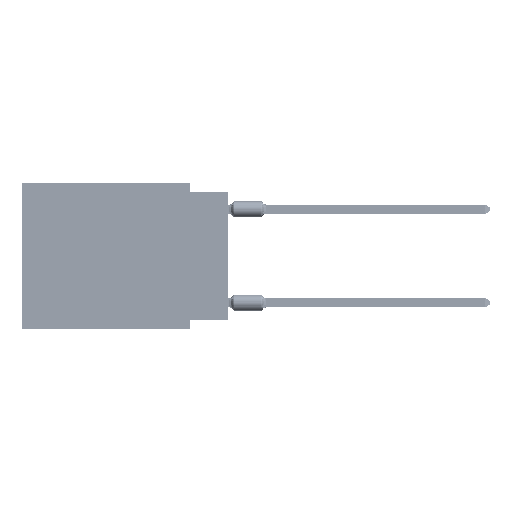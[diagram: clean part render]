
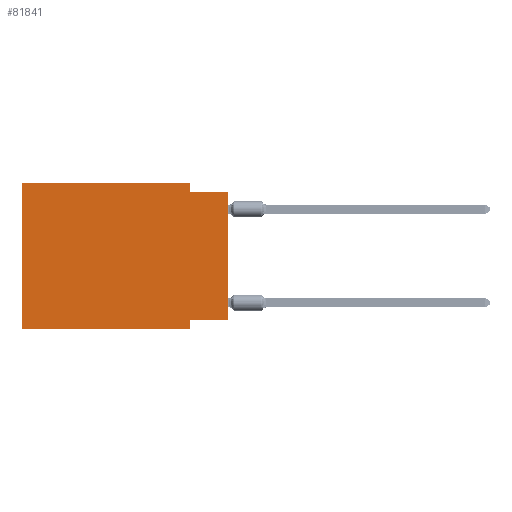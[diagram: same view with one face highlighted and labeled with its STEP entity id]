
A CAD part, left-side view. The second image highlights one B-rep face of the part: STEP entity #81841.
In plain terms, the highlighted planar face has unit normal (-1, 0, 0).
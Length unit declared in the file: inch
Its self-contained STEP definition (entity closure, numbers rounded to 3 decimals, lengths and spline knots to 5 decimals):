
#210 = LINE ( 'NONE', #67478, #28942 ) ;
#4783 = CARTESIAN_POINT ( 'NONE',  ( 0., 0.1, 0. ) ) ;
#5134 = EDGE_CURVE ( 'NONE', #66802, #17737, #49236, .T. ) ;
#6592 = DIRECTION ( 'NONE',  ( 0., 0., -1. ) ) ;
#6637 = VECTOR ( 'NONE', #6592, 39.37008 ) ;
#8726 = VERTEX_POINT ( 'NONE', #70090 ) ;
#9835 = AXIS2_PLACEMENT_3D ( 'NONE', #36340, #56525, #29174 ) ;
#14161 = DIRECTION ( 'NONE',  ( 0., -1., 0. ) ) ;
#15263 = FACE_OUTER_BOUND ( 'NONE', #15347, .T. ) ;
#15347 = EDGE_LOOP ( 'NONE', ( #36349, #33733, #61894, #77230, #71015, #83137, #86440, #34838 ) ) ;
#16062 = VERTEX_POINT ( 'NONE', #21957 ) ;
#17737 = VERTEX_POINT ( 'NONE', #36711 ) ;
#17960 = LINE ( 'NONE', #51176, #39999 ) ;
#20198 = DIRECTION ( 'NONE',  ( 0., -1., 0. ) ) ;
#20569 = CARTESIAN_POINT ( 'NONE',  ( 0., 0., -0.365 ) ) ;
#21957 = CARTESIAN_POINT ( 'NONE',  ( 0., 0., -0.365 ) ) ;
#26062 = LINE ( 'NONE', #67277, #36022 ) ;
#28281 = VECTOR ( 'NONE', #14161, 39.37008 ) ;
#28587 = DIRECTION ( 'NONE',  ( 0., 0., 1. ) ) ;
#28942 = VECTOR ( 'NONE', #47772, 39.37008 ) ;
#29174 = DIRECTION ( 'NONE',  ( 0., 0., -1. ) ) ;
#31459 = VERTEX_POINT ( 'NONE', #50695 ) ;
#32402 = CARTESIAN_POINT ( 'NONE',  ( 0., 0., -0.025 ) ) ;
#33261 = EDGE_CURVE ( 'NONE', #17737, #31459, #67974, .T. ) ;
#33515 = VERTEX_POINT ( 'NONE', #32402 ) ;
#33733 = ORIENTED_EDGE ( 'NONE', *, *, #40200, .F. ) ;
#34273 = CARTESIAN_POINT ( 'NONE',  ( 0., 0.55, -0.39 ) ) ;
#34436 = CARTESIAN_POINT ( 'NONE',  ( 0., 0.1, -0.39 ) ) ;
#34838 = ORIENTED_EDGE ( 'NONE', *, *, #75110, .F. ) ;
#36022 = VECTOR ( 'NONE', #20198, 39.37008 ) ;
#36340 = CARTESIAN_POINT ( 'NONE',  ( 0., 0.55, 0. ) ) ;
#36349 = ORIENTED_EDGE ( 'NONE', *, *, #38085, .T. ) ;
#36711 = CARTESIAN_POINT ( 'NONE',  ( 0., 0.55, 0. ) ) ;
#38085 = EDGE_CURVE ( 'NONE', #16062, #33515, #210, .T. ) ;
#39011 = CARTESIAN_POINT ( 'NONE',  ( 0., 0.1, -0.025 ) ) ;
#39999 = VECTOR ( 'NONE', #87417, 39.37008 ) ;
#40200 = EDGE_CURVE ( 'NONE', #45737, #33515, #26062, .T. ) ;
#44770 = DIRECTION ( 'NONE',  ( 0., 0., -1. ) ) ;
#45737 = VERTEX_POINT ( 'NONE', #39011 ) ;
#47772 = DIRECTION ( 'NONE',  ( 0., 0., 1. ) ) ;
#48720 = CARTESIAN_POINT ( 'NONE',  ( 0., 0.55, 0. ) ) ;
#49236 = LINE ( 'NONE', #76986, #67402 ) ;
#50695 = CARTESIAN_POINT ( 'NONE',  ( 0., 0.1, 0. ) ) ;
#51176 = CARTESIAN_POINT ( 'NONE',  ( 0., 0.55, -0.39 ) ) ;
#52433 = EDGE_CURVE ( 'NONE', #75968, #8726, #55484, .T. ) ;
#55484 = LINE ( 'NONE', #34436, #6637 ) ;
#56525 = DIRECTION ( 'NONE',  ( 1., 0., 0. ) ) ;
#56612 = VECTOR ( 'NONE', #44770, 39.37008 ) ;
#57288 = EDGE_CURVE ( 'NONE', #66802, #8726, #17960, .T. ) ;
#60546 = LINE ( 'NONE', #20569, #72270 ) ;
#61756 = EDGE_CURVE ( 'NONE', #31459, #45737, #66237, .T. ) ;
#61894 = ORIENTED_EDGE ( 'NONE', *, *, #61756, .F. ) ;
#62368 = CARTESIAN_POINT ( 'NONE',  ( 0., 0.1, -0.365 ) ) ;
#66237 = LINE ( 'NONE', #4783, #56612 ) ;
#66802 = VERTEX_POINT ( 'NONE', #34273 ) ;
#67277 = CARTESIAN_POINT ( 'NONE',  ( 0., 0., -0.025 ) ) ;
#67402 = VECTOR ( 'NONE', #28587, 39.37008 ) ;
#67478 = CARTESIAN_POINT ( 'NONE',  ( 0., 0., 0. ) ) ;
#67974 = LINE ( 'NONE', #48720, #28281 ) ;
#70090 = CARTESIAN_POINT ( 'NONE',  ( 0., 0.1, -0.39 ) ) ;
#71015 = ORIENTED_EDGE ( 'NONE', *, *, #5134, .F. ) ;
#72270 = VECTOR ( 'NONE', #74820, 39.37008 ) ;
#74820 = DIRECTION ( 'NONE',  ( 0., 1., 0. ) ) ;
#75110 = EDGE_CURVE ( 'NONE', #16062, #75968, #60546, .T. ) ;
#75968 = VERTEX_POINT ( 'NONE', #62368 ) ;
#76986 = CARTESIAN_POINT ( 'NONE',  ( 0., 0.55, 0. ) ) ;
#77230 = ORIENTED_EDGE ( 'NONE', *, *, #33261, .F. ) ;
#81841 = ADVANCED_FACE ( 'NONE', ( #15263 ), #83855, .F. ) ;
#83137 = ORIENTED_EDGE ( 'NONE', *, *, #57288, .T. ) ;
#83855 = PLANE ( 'NONE',  #9835 ) ;
#86440 = ORIENTED_EDGE ( 'NONE', *, *, #52433, .F. ) ;
#87417 = DIRECTION ( 'NONE',  ( 0., -1., 0. ) ) ;
